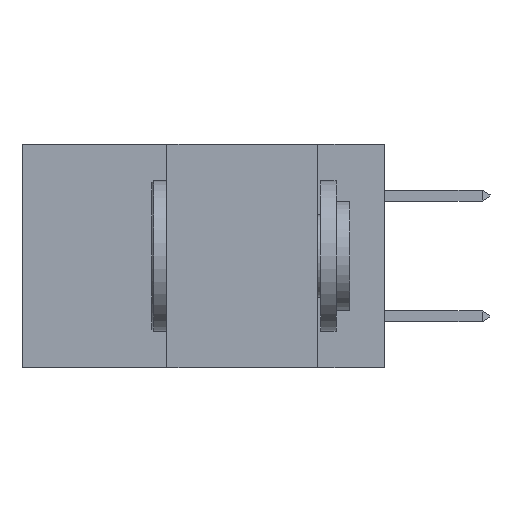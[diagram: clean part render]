
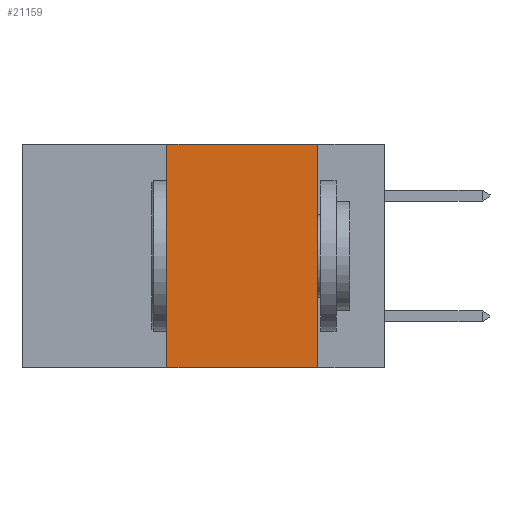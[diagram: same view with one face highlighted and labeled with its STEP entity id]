
A CAD part, left-side view. The second image highlights one B-rep face of the part: STEP entity #21159.
In plain terms, the highlighted planar face has unit normal (-1, 0, 0).
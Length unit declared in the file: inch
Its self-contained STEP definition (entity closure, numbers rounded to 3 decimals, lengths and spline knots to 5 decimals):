
#1186 = DIRECTION ( 'NONE',  ( 0., 0., -1. ) ) ;
#4773 = VERTEX_POINT ( 'NONE', #20188 ) ;
#5629 = VECTOR ( 'NONE', #7833, 39.37008 ) ;
#6245 = VERTEX_POINT ( 'NONE', #13267 ) ;
#6269 = ORIENTED_EDGE ( 'NONE', *, *, #17481, .F. ) ;
#6849 = ORIENTED_EDGE ( 'NONE', *, *, #18476, .F. ) ;
#7109 = CARTESIAN_POINT ( 'NONE',  ( 0., 0.6, 0. ) ) ;
#7799 = ORIENTED_EDGE ( 'NONE', *, *, #22320, .F. ) ;
#7833 = DIRECTION ( 'NONE',  ( 0., -1., 0. ) ) ;
#7996 = CARTESIAN_POINT ( 'NONE',  ( 0., 0.6, 0. ) ) ;
#8599 = CARTESIAN_POINT ( 'NONE',  ( 0., 0.11, -0.37 ) ) ;
#9650 = LINE ( 'NONE', #18681, #14671 ) ;
#10943 = EDGE_LOOP ( 'NONE', ( #6849, #6269, #7799, #35854 ) ) ;
#13267 = CARTESIAN_POINT ( 'NONE',  ( 0., 0.11, 0. ) ) ;
#13939 = DIRECTION ( 'NONE',  ( 0., -1., 0. ) ) ;
#14671 = VECTOR ( 'NONE', #28716, 39.37008 ) ;
#17129 = DIRECTION ( 'NONE',  ( 0., 0., -1. ) ) ;
#17481 = EDGE_CURVE ( 'NONE', #4773, #6245, #37409, .T. ) ;
#18476 = EDGE_CURVE ( 'NONE', #6245, #35939, #39905, .T. ) ;
#18681 = CARTESIAN_POINT ( 'NONE',  ( 0., 0.36, 0. ) ) ;
#20188 = CARTESIAN_POINT ( 'NONE',  ( 0., 0.36, 0. ) ) ;
#20739 = CARTESIAN_POINT ( 'NONE',  ( 0., 0.11, 0. ) ) ;
#21159 = ADVANCED_FACE ( 'NONE', ( #23614 ), #29745, .F. ) ;
#22056 = AXIS2_PLACEMENT_3D ( 'NONE', #7109, #32840, #1186 ) ;
#22320 = EDGE_CURVE ( 'NONE', #27584, #4773, #9650, .T. ) ;
#23614 = FACE_OUTER_BOUND ( 'NONE', #10943, .T. ) ;
#26109 = EDGE_CURVE ( 'NONE', #27584, #35939, #31190, .T. ) ;
#27584 = VERTEX_POINT ( 'NONE', #37229 ) ;
#27704 = VECTOR ( 'NONE', #13939, 39.37008 ) ;
#28716 = DIRECTION ( 'NONE',  ( 0., 0., 1. ) ) ;
#29745 = PLANE ( 'NONE',  #22056 ) ;
#31190 = LINE ( 'NONE', #36757, #27704 ) ;
#32840 = DIRECTION ( 'NONE',  ( 1., 0., 0. ) ) ;
#35854 = ORIENTED_EDGE ( 'NONE', *, *, #26109, .T. ) ;
#35939 = VERTEX_POINT ( 'NONE', #8599 ) ;
#36757 = CARTESIAN_POINT ( 'NONE',  ( 0., 0.6, -0.37 ) ) ;
#37229 = CARTESIAN_POINT ( 'NONE',  ( 0., 0.36, -0.37 ) ) ;
#37376 = VECTOR ( 'NONE', #17129, 39.37008 ) ;
#37409 = LINE ( 'NONE', #7996, #5629 ) ;
#39905 = LINE ( 'NONE', #20739, #37376 ) ;
